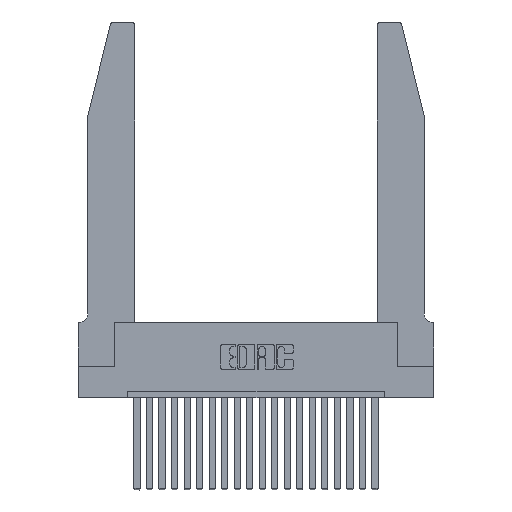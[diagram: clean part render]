
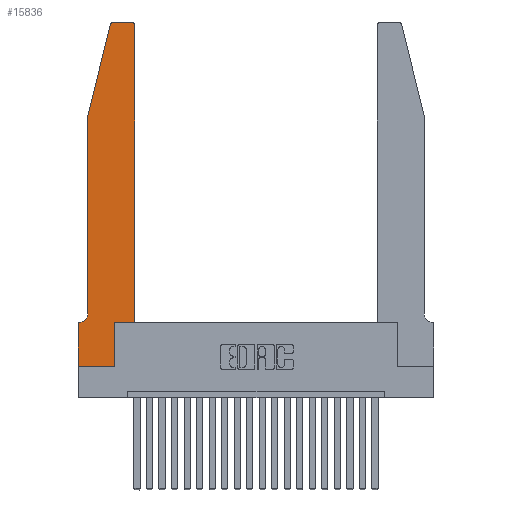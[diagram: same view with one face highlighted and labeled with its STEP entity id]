
A CAD part, top view. The second image highlights one B-rep face of the part: STEP entity #15836.
In plain terms, the highlighted planar face has unit normal (0, 0, 1).
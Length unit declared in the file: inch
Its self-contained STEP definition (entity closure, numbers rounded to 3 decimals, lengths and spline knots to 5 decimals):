
#107 = VECTOR ( 'NONE', #17170, 39.37008 ) ;
#142 = VERTEX_POINT ( 'NONE', #21862 ) ;
#211 = CIRCLE ( 'NONE', #20288, 0.03 ) ;
#213 = CARTESIAN_POINT ( 'NONE',  ( 0.0755, 2., 0.37 ) ) ;
#283 = CARTESIAN_POINT ( 'NONE',  ( 0.2865, 0.35, 0.37 ) ) ;
#514 = CARTESIAN_POINT ( 'NONE',  ( 0.4205, 2.75, 0.37 ) ) ;
#592 = VERTEX_POINT ( 'NONE', #514 ) ;
#653 = CARTESIAN_POINT ( 'NONE',  ( 0.2605, 2.75, 0.37 ) ) ;
#655 = ORIENTED_EDGE ( 'NONE', *, *, #6362, .T. ) ;
#985 = CARTESIAN_POINT ( 'NONE',  ( 0.0755, 0.42, 0.37 ) ) ;
#1161 = CARTESIAN_POINT ( 'NONE',  ( 0., 0., 0.37 ) ) ;
#1324 = ORIENTED_EDGE ( 'NONE', *, *, #10539, .T. ) ;
#1498 = EDGE_CURVE ( 'NONE', #11138, #142, #10592, .T. ) ;
#1596 = EDGE_CURVE ( 'NONE', #21935, #2001, #17959, .T. ) ;
#1874 = CARTESIAN_POINT ( 'NONE',  ( 0., 0., 0.37 ) ) ;
#2001 = VERTEX_POINT ( 'NONE', #20624 ) ;
#2025 = EDGE_CURVE ( 'NONE', #14918, #592, #211, .T. ) ;
#2225 = CARTESIAN_POINT ( 'NONE',  ( 0.284, 2.75, 0.37 ) ) ;
#2698 = AXIS2_PLACEMENT_3D ( 'NONE', #5571, #11345, #6169 ) ;
#2720 = ORIENTED_EDGE ( 'NONE', *, *, #10854, .T. ) ;
#2880 = VECTOR ( 'NONE', #6599, 39.37008 ) ;
#3193 = DIRECTION ( 'NONE',  ( 0., 0., 1. ) ) ;
#3271 = CARTESIAN_POINT ( 'NONE',  ( 0.4205, 2.72, 0.37 ) ) ;
#3329 = CARTESIAN_POINT ( 'NONE',  ( 0.4505, 0.35, 0.37 ) ) ;
#3473 = CARTESIAN_POINT ( 'NONE',  ( 0.4505, 0.35, 0.37 ) ) ;
#3605 = VERTEX_POINT ( 'NONE', #985 ) ;
#4099 = ORIENTED_EDGE ( 'NONE', *, *, #11462, .T. ) ;
#4911 = DIRECTION ( 'NONE',  ( 1., 0., 0. ) ) ;
#4922 = DIRECTION ( 'NONE',  ( 0., 1., 0. ) ) ;
#5069 = EDGE_LOOP ( 'NONE', ( #11407, #5336, #18277, #8988, #17284, #16685, #1324, #655, #9590, #4099, #2720, #19520 ) ) ;
#5336 = ORIENTED_EDGE ( 'NONE', *, *, #10037, .T. ) ;
#5571 = CARTESIAN_POINT ( 'NONE',  ( 0.0055, 0.42, 0.37 ) ) ;
#5688 = LINE ( 'NONE', #11496, #11123 ) ;
#6169 = DIRECTION ( 'NONE',  ( -1., 0., 0. ) ) ;
#6221 = AXIS2_PLACEMENT_3D ( 'NONE', #12317, #8807, #22593 ) ;
#6362 = EDGE_CURVE ( 'NONE', #13669, #11138, #15568, .T. ) ;
#6599 = DIRECTION ( 'NONE',  ( 1., 0., 0. ) ) ;
#6740 = LINE ( 'NONE', #653, #11359 ) ;
#6782 = VECTOR ( 'NONE', #21088, 39.37008 ) ;
#7177 = DIRECTION ( 'NONE',  ( 0., 1., 0. ) ) ;
#7262 = VERTEX_POINT ( 'NONE', #3473 ) ;
#7565 = LINE ( 'NONE', #3329, #2880 ) ;
#7902 = VECTOR ( 'NONE', #21870, 39.37008 ) ;
#8807 = DIRECTION ( 'NONE',  ( 0., 0., 1. ) ) ;
#8988 = ORIENTED_EDGE ( 'NONE', *, *, #8997, .T. ) ;
#8997 = EDGE_CURVE ( 'NONE', #2001, #3605, #21259, .T. ) ;
#9021 = DIRECTION ( 'NONE',  ( 1., 0., 0. ) ) ;
#9463 = AXIS2_PLACEMENT_3D ( 'NONE', #13023, #3193, #4911 ) ;
#9590 = ORIENTED_EDGE ( 'NONE', *, *, #1498, .T. ) ;
#9876 = CARTESIAN_POINT ( 'NONE',  ( 0.0055, 0.35, 0.37 ) ) ;
#10037 = EDGE_CURVE ( 'NONE', #20239, #21935, #15265, .T. ) ;
#10340 = DIRECTION ( 'NONE',  ( 0., 0., 1. ) ) ;
#10539 = EDGE_CURVE ( 'NONE', #15422, #13669, #20125, .T. ) ;
#10592 = LINE ( 'NONE', #283, #13624 ) ;
#10599 = DIRECTION ( 'NONE',  ( -0.239, -0.971, 0. ) ) ;
#10854 = EDGE_CURVE ( 'NONE', #7262, #14918, #5688, .T. ) ;
#11123 = VECTOR ( 'NONE', #4922, 39.37008 ) ;
#11138 = VERTEX_POINT ( 'NONE', #18040 ) ;
#11324 = EDGE_CURVE ( 'NONE', #592, #20239, #6740, .T. ) ;
#11345 = DIRECTION ( 'NONE',  ( 0., 0., -1. ) ) ;
#11359 = VECTOR ( 'NONE', #19853, 39.37008 ) ;
#11407 = ORIENTED_EDGE ( 'NONE', *, *, #11324, .T. ) ;
#11462 = EDGE_CURVE ( 'NONE', #142, #7262, #7565, .T. ) ;
#11496 = CARTESIAN_POINT ( 'NONE',  ( 0.4505, 0.35, 0.37 ) ) ;
#11871 = DIRECTION ( 'NONE',  ( 1., 0., 0. ) ) ;
#12317 = CARTESIAN_POINT ( 'NONE',  ( 0., 0.35, 0.37 ) ) ;
#12686 = LINE ( 'NONE', #20830, #107 ) ;
#13023 = CARTESIAN_POINT ( 'NONE',  ( 0.284, 2.72, 0.37 ) ) ;
#13624 = VECTOR ( 'NONE', #7177, 39.37008 ) ;
#13669 = VERTEX_POINT ( 'NONE', #1161 ) ;
#14918 = VERTEX_POINT ( 'NONE', #21733 ) ;
#15087 = CARTESIAN_POINT ( 'NONE',  ( 0., 0.35, 0.37 ) ) ;
#15265 = CIRCLE ( 'NONE', #9463, 0.03 ) ;
#15422 = VERTEX_POINT ( 'NONE', #15087 ) ;
#15568 = LINE ( 'NONE', #18977, #17205 ) ;
#15581 = PLANE ( 'NONE',  #6221 ) ;
#15836 = ADVANCED_FACE ( 'NONE', ( #16819 ), #15581, .T. ) ;
#16685 = ORIENTED_EDGE ( 'NONE', *, *, #17443, .T. ) ;
#16819 = FACE_OUTER_BOUND ( 'NONE', #5069, .T. ) ;
#17170 = DIRECTION ( 'NONE',  ( -1., 0., 0. ) ) ;
#17205 = VECTOR ( 'NONE', #9021, 39.37008 ) ;
#17284 = ORIENTED_EDGE ( 'NONE', *, *, #17597, .T. ) ;
#17443 = EDGE_CURVE ( 'NONE', #22219, #15422, #12686, .T. ) ;
#17597 = EDGE_CURVE ( 'NONE', #3605, #22219, #19203, .T. ) ;
#17959 = LINE ( 'NONE', #213, #18769 ) ;
#18040 = CARTESIAN_POINT ( 'NONE',  ( 0.2865, 0., 0.37 ) ) ;
#18277 = ORIENTED_EDGE ( 'NONE', *, *, #1596, .T. ) ;
#18748 = CARTESIAN_POINT ( 'NONE',  ( 0.0755, 2., 0.37 ) ) ;
#18769 = VECTOR ( 'NONE', #10599, 39.37008 ) ;
#18977 = CARTESIAN_POINT ( 'NONE',  ( 0., 0., 0.37 ) ) ;
#19173 = CARTESIAN_POINT ( 'NONE',  ( 0.25487, 2.72718, 0.37 ) ) ;
#19203 = CIRCLE ( 'NONE', #2698, 0.07 ) ;
#19520 = ORIENTED_EDGE ( 'NONE', *, *, #2025, .T. ) ;
#19853 = DIRECTION ( 'NONE',  ( -1., 0., 0. ) ) ;
#20125 = LINE ( 'NONE', #1874, #6782 ) ;
#20239 = VERTEX_POINT ( 'NONE', #2225 ) ;
#20288 = AXIS2_PLACEMENT_3D ( 'NONE', #3271, #10340, #11871 ) ;
#20624 = CARTESIAN_POINT ( 'NONE',  ( 0.0755, 2., 0.37 ) ) ;
#20830 = CARTESIAN_POINT ( 'NONE',  ( 0.0755, 0.35, 0.37 ) ) ;
#21088 = DIRECTION ( 'NONE',  ( 0., -1., 0. ) ) ;
#21259 = LINE ( 'NONE', #18748, #7902 ) ;
#21733 = CARTESIAN_POINT ( 'NONE',  ( 0.4505, 2.72, 0.37 ) ) ;
#21862 = CARTESIAN_POINT ( 'NONE',  ( 0.2865, 0.35, 0.37 ) ) ;
#21870 = DIRECTION ( 'NONE',  ( 0., -1., 0. ) ) ;
#21935 = VERTEX_POINT ( 'NONE', #19173 ) ;
#22219 = VERTEX_POINT ( 'NONE', #9876 ) ;
#22593 = DIRECTION ( 'NONE',  ( 1., 0., 0. ) ) ;
